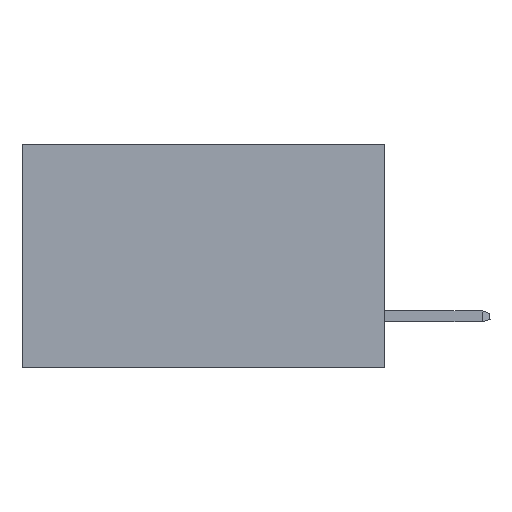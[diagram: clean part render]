
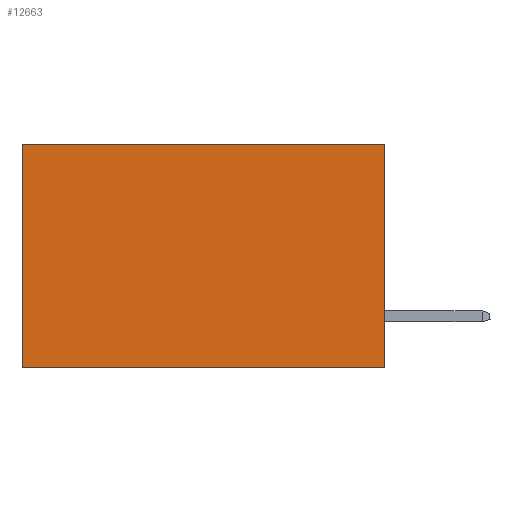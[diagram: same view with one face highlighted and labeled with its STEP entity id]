
A CAD part, left-side view. The second image highlights one B-rep face of the part: STEP entity #12663.
In plain terms, the highlighted planar face has unit normal (-1, 0, 0).
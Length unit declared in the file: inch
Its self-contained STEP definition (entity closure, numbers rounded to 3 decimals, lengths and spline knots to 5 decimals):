
#100 = VERTEX_POINT ( 'NONE', #4381 ) ;
#191 = CARTESIAN_POINT ( 'NONE',  ( 0.298, 0.6, 0. ) ) ;
#234 = LINE ( 'NONE', #642, #5457 ) ;
#642 = CARTESIAN_POINT ( 'NONE',  ( 0.298, 0., 0. ) ) ;
#1400 = VECTOR ( 'NONE', #9394, 39.37008 ) ;
#1597 = DIRECTION ( 'NONE',  ( 0., 0., -1. ) ) ;
#1654 = VERTEX_POINT ( 'NONE', #5818 ) ;
#1977 = DIRECTION ( 'NONE',  ( 1., 0., 0. ) ) ;
#2457 = EDGE_CURVE ( 'NONE', #100, #9955, #234, .T. ) ;
#2767 = ORIENTED_EDGE ( 'NONE', *, *, #2457, .T. ) ;
#2976 = VECTOR ( 'NONE', #6834, 39.37008 ) ;
#3057 = CARTESIAN_POINT ( 'NONE',  ( 0.298, 0.6, -0.37 ) ) ;
#3261 = CARTESIAN_POINT ( 'NONE',  ( 0.298, 0., 0. ) ) ;
#3428 = AXIS2_PLACEMENT_3D ( 'NONE', #7034, #1977, #10083 ) ;
#4289 = LINE ( 'NONE', #3261, #12147 ) ;
#4381 = CARTESIAN_POINT ( 'NONE',  ( 0.298, 0., 0. ) ) ;
#4385 = LINE ( 'NONE', #11978, #2976 ) ;
#5047 = PLANE ( 'NONE',  #3428 ) ;
#5282 = EDGE_CURVE ( 'NONE', #100, #1654, #4289, .T. ) ;
#5457 = VECTOR ( 'NONE', #6647, 39.37008 ) ;
#5818 = CARTESIAN_POINT ( 'NONE',  ( 0.298, 0., -0.37 ) ) ;
#6003 = ORIENTED_EDGE ( 'NONE', *, *, #8120, .T. ) ;
#6578 = EDGE_LOOP ( 'NONE', ( #6003, #10442, #7156, #2767 ) ) ;
#6647 = DIRECTION ( 'NONE',  ( 0., 1., 0. ) ) ;
#6798 = LINE ( 'NONE', #191, #1400 ) ;
#6831 = FACE_OUTER_BOUND ( 'NONE', #6578, .T. ) ;
#6834 = DIRECTION ( 'NONE',  ( 0., 1., 0. ) ) ;
#7034 = CARTESIAN_POINT ( 'NONE',  ( 0.298, 0., 0. ) ) ;
#7156 = ORIENTED_EDGE ( 'NONE', *, *, #5282, .F. ) ;
#7458 = EDGE_CURVE ( 'NONE', #1654, #12654, #4385, .T. ) ;
#8120 = EDGE_CURVE ( 'NONE', #9955, #12654, #6798, .T. ) ;
#9394 = DIRECTION ( 'NONE',  ( 0., 0., -1. ) ) ;
#9955 = VERTEX_POINT ( 'NONE', #10696 ) ;
#10083 = DIRECTION ( 'NONE',  ( 0., 0., -1. ) ) ;
#10442 = ORIENTED_EDGE ( 'NONE', *, *, #7458, .F. ) ;
#10696 = CARTESIAN_POINT ( 'NONE',  ( 0.298, 0.6, 0. ) ) ;
#11978 = CARTESIAN_POINT ( 'NONE',  ( 0.298, 0., -0.37 ) ) ;
#12147 = VECTOR ( 'NONE', #1597, 39.37008 ) ;
#12654 = VERTEX_POINT ( 'NONE', #3057 ) ;
#12663 = ADVANCED_FACE ( 'NONE', ( #6831 ), #5047, .F. ) ;
